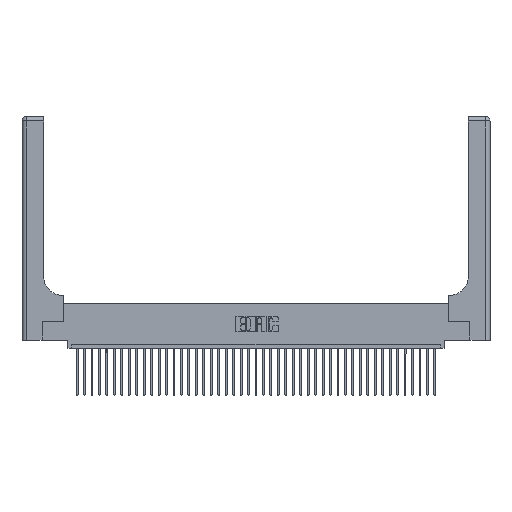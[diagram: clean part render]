
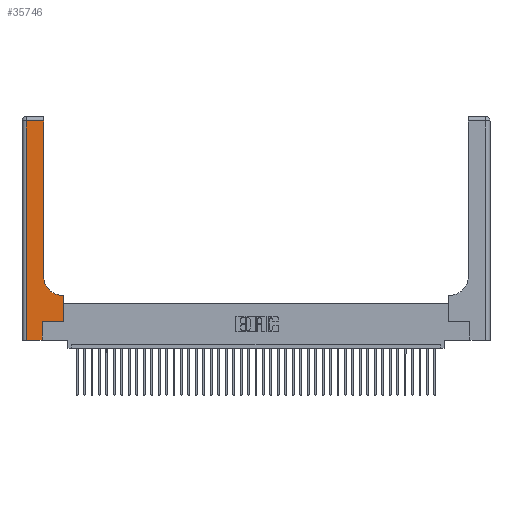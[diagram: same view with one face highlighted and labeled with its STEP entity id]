
A CAD part, top view. The second image highlights one B-rep face of the part: STEP entity #35746.
In plain terms, the highlighted planar face has unit normal (0, 0, 1).
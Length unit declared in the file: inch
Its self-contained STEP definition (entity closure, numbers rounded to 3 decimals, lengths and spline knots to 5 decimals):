
#360 = CARTESIAN_POINT ( 'NONE',  ( 0.2915, 0.6, 0.37 ) ) ;
#504 = DIRECTION ( 'NONE',  ( -1., 0., 0. ) ) ;
#823 = LINE ( 'NONE', #360, #20812 ) ;
#941 = CARTESIAN_POINT ( 'NONE',  ( 0., 3., 0.37 ) ) ;
#1394 = PLANE ( 'NONE',  #31097 ) ;
#1584 = CARTESIAN_POINT ( 'NONE',  ( 0.06, 3., 0.37 ) ) ;
#1595 = VECTOR ( 'NONE', #35212, 39.37008 ) ;
#1800 = CARTESIAN_POINT ( 'NONE',  ( 0.269, 0., 0.37 ) ) ;
#2453 = ORIENTED_EDGE ( 'NONE', *, *, #35173, .T. ) ;
#2681 = DIRECTION ( 'NONE',  ( 0., 0., -1. ) ) ;
#2824 = CIRCLE ( 'NONE', #40538, 0.25 ) ;
#3838 = ORIENTED_EDGE ( 'NONE', *, *, #12166, .T. ) ;
#3935 = DIRECTION ( 'NONE',  ( 0., 1., 0. ) ) ;
#4538 = EDGE_CURVE ( 'NONE', #8117, #41161, #37709, .T. ) ;
#5025 = CARTESIAN_POINT ( 'NONE',  ( 0.06, 0., 0.37 ) ) ;
#5256 = CARTESIAN_POINT ( 'NONE',  ( 0.5415, 0.6, 0.37 ) ) ;
#6155 = DIRECTION ( 'NONE',  ( 1., 0., 0. ) ) ;
#6671 = ORIENTED_EDGE ( 'NONE', *, *, #38736, .T. ) ;
#7676 = VERTEX_POINT ( 'NONE', #29933 ) ;
#7775 = LINE ( 'NONE', #10451, #31186 ) ;
#8117 = VERTEX_POINT ( 'NONE', #37676 ) ;
#9333 = VERTEX_POINT ( 'NONE', #24744 ) ;
#10017 = LINE ( 'NONE', #32436, #1595 ) ;
#10042 = CARTESIAN_POINT ( 'NONE',  ( 0.269, 0.25, 0.37 ) ) ;
#10451 = CARTESIAN_POINT ( 'NONE',  ( 0.269, 0., 0.37 ) ) ;
#10938 = ORIENTED_EDGE ( 'NONE', *, *, #4538, .T. ) ;
#12166 = EDGE_CURVE ( 'NONE', #38043, #15987, #2824, .T. ) ;
#12993 = VERTEX_POINT ( 'NONE', #1800 ) ;
#13365 = VECTOR ( 'NONE', #34008, 39.37008 ) ;
#13818 = ORIENTED_EDGE ( 'NONE', *, *, #20877, .T. ) ;
#13868 = LINE ( 'NONE', #23981, #13365 ) ;
#13876 = LINE ( 'NONE', #16565, #31325 ) ;
#15987 = VERTEX_POINT ( 'NONE', #36066 ) ;
#16565 = CARTESIAN_POINT ( 'NONE',  ( 0.5585, 0.25, 0.37 ) ) ;
#16894 = ORIENTED_EDGE ( 'NONE', *, *, #25735, .T. ) ;
#16992 = CARTESIAN_POINT ( 'NONE',  ( 0.5585, 0.25, 0.37 ) ) ;
#18186 = ORIENTED_EDGE ( 'NONE', *, *, #38213, .T. ) ;
#18644 = DIRECTION ( 'NONE',  ( 1., 0., 0. ) ) ;
#20739 = VECTOR ( 'NONE', #27057, 39.37008 ) ;
#20812 = VECTOR ( 'NONE', #504, 39.37008 ) ;
#20877 = EDGE_CURVE ( 'NONE', #41161, #12993, #10017, .T. ) ;
#22865 = EDGE_CURVE ( 'NONE', #7676, #33311, #30792, .T. ) ;
#23002 = LINE ( 'NONE', #31120, #39461 ) ;
#23667 = DIRECTION ( 'NONE',  ( -1., 0., 0. ) ) ;
#23981 = CARTESIAN_POINT ( 'NONE',  ( 0., 2.94, 0.37 ) ) ;
#24744 = CARTESIAN_POINT ( 'NONE',  ( 0.5585, 0.6, 0.37 ) ) ;
#25735 = EDGE_CURVE ( 'NONE', #29149, #8117, #13868, .T. ) ;
#26777 = VECTOR ( 'NONE', #18644, 39.37008 ) ;
#27057 = DIRECTION ( 'NONE',  ( 0., -1., 0. ) ) ;
#27215 = FACE_OUTER_BOUND ( 'NONE', #40306, .T. ) ;
#27893 = ORIENTED_EDGE ( 'NONE', *, *, #31725, .T. ) ;
#28691 = CARTESIAN_POINT ( 'NONE',  ( 0.2915, 2.94, 0.37 ) ) ;
#29149 = VERTEX_POINT ( 'NONE', #28691 ) ;
#29933 = CARTESIAN_POINT ( 'NONE',  ( 0.269, 0.25, 0.37 ) ) ;
#30792 = LINE ( 'NONE', #10042, #26777 ) ;
#31097 = AXIS2_PLACEMENT_3D ( 'NONE', #941, #35885, #23667 ) ;
#31120 = CARTESIAN_POINT ( 'NONE',  ( 0.2915, 3., 0.37 ) ) ;
#31186 = VECTOR ( 'NONE', #3935, 39.37008 ) ;
#31325 = VECTOR ( 'NONE', #38888, 39.37008 ) ;
#31725 = EDGE_CURVE ( 'NONE', #15987, #29149, #23002, .T. ) ;
#32436 = CARTESIAN_POINT ( 'NONE',  ( 0., 0., 0.37 ) ) ;
#32441 = ORIENTED_EDGE ( 'NONE', *, *, #22865, .T. ) ;
#33311 = VERTEX_POINT ( 'NONE', #16992 ) ;
#34008 = DIRECTION ( 'NONE',  ( -1., 0., 0. ) ) ;
#35173 = EDGE_CURVE ( 'NONE', #12993, #7676, #7775, .T. ) ;
#35212 = DIRECTION ( 'NONE',  ( 1., 0., 0. ) ) ;
#35746 = ADVANCED_FACE ( 'NONE', ( #27215 ), #1394, .F. ) ;
#35885 = DIRECTION ( 'NONE',  ( 0., 0., -1. ) ) ;
#36066 = CARTESIAN_POINT ( 'NONE',  ( 0.2915, 0.85, 0.37 ) ) ;
#37613 = CARTESIAN_POINT ( 'NONE',  ( 0.5415, 0.85, 0.37 ) ) ;
#37676 = CARTESIAN_POINT ( 'NONE',  ( 0.06, 2.94, 0.37 ) ) ;
#37709 = LINE ( 'NONE', #1584, #20739 ) ;
#38043 = VERTEX_POINT ( 'NONE', #5256 ) ;
#38213 = EDGE_CURVE ( 'NONE', #33311, #9333, #13876, .T. ) ;
#38736 = EDGE_CURVE ( 'NONE', #9333, #38043, #823, .T. ) ;
#38888 = DIRECTION ( 'NONE',  ( 0., 1., 0. ) ) ;
#39461 = VECTOR ( 'NONE', #40883, 39.37008 ) ;
#40306 = EDGE_LOOP ( 'NONE', ( #27893, #16894, #10938, #13818, #2453, #32441, #18186, #6671, #3838 ) ) ;
#40538 = AXIS2_PLACEMENT_3D ( 'NONE', #37613, #2681, #6155 ) ;
#40883 = DIRECTION ( 'NONE',  ( 0., 1., 0. ) ) ;
#41161 = VERTEX_POINT ( 'NONE', #5025 ) ;
